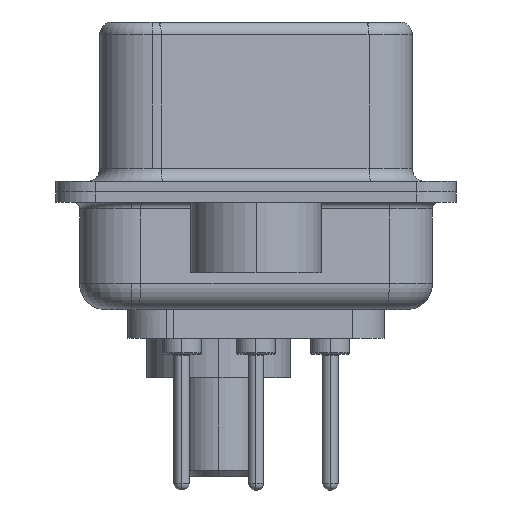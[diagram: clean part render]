
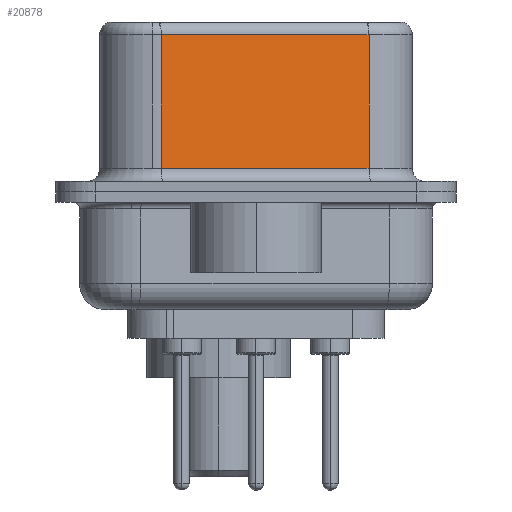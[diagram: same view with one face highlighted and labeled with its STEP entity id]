
A CAD part, left-side view. The second image highlights one B-rep face of the part: STEP entity #20878.
In plain terms, the highlighted planar face has unit normal (-0.985, -0.174, 0).
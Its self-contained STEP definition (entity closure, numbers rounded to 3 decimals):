
#35 = CARTESIAN_POINT ( 'NONE',  ( 5.132, -4.322, 0.9 ) ) ;
#919 = CARTESIAN_POINT ( 'NONE',  ( 5.132, -4.322, 6.52 ) ) ;
#1371 = LINE ( 'NONE', #1636, #23242 ) ;
#1636 = CARTESIAN_POINT ( 'NONE',  ( 5.132, -4.322, 6.02 ) ) ;
#1739 = VECTOR ( 'NONE', #6403, 1000. ) ;
#1904 = EDGE_CURVE ( 'NONE', #24573, #15131, #2415, .T. ) ;
#2415 = LINE ( 'NONE', #919, #1739 ) ;
#3811 = ORIENTED_EDGE ( 'NONE', *, *, #1904, .F. ) ;
#3835 = DIRECTION ( 'NONE',  ( -0.174, 0.985, 0. ) ) ;
#6403 = DIRECTION ( 'NONE',  ( 0., 0., -1. ) ) ;
#6709 = VERTEX_POINT ( 'NONE', #12838 ) ;
#6883 = CARTESIAN_POINT ( 'NONE',  ( 3.73, 3.628, 6.02 ) ) ;
#10946 = LINE ( 'NONE', #35, #27660 ) ;
#11010 = CARTESIAN_POINT ( 'NONE',  ( 3.73, 3.628, 6.52 ) ) ;
#11088 = CARTESIAN_POINT ( 'NONE',  ( 5.132, -4.322, 0.9 ) ) ;
#11819 = EDGE_CURVE ( 'NONE', #24573, #27920, #1371, .T. ) ;
#12649 = DIRECTION ( 'NONE',  ( 0.985, 0.174, 0. ) ) ;
#12838 = CARTESIAN_POINT ( 'NONE',  ( 3.73, 3.628, 0.9 ) ) ;
#13059 = LINE ( 'NONE', #11010, #23986 ) ;
#15131 = VERTEX_POINT ( 'NONE', #11088 ) ;
#17883 = EDGE_LOOP ( 'NONE', ( #3811, #19255, #24716, #22325 ) ) ;
#19084 = EDGE_CURVE ( 'NONE', #27920, #6709, #13059, .T. ) ;
#19255 = ORIENTED_EDGE ( 'NONE', *, *, #11819, .T. ) ;
#19712 = DIRECTION ( 'NONE',  ( 0., 0., -1. ) ) ;
#20878 = ADVANCED_FACE ( 'NONE', ( #22548 ), #23600, .F. ) ;
#21446 = CARTESIAN_POINT ( 'NONE',  ( 5.132, -4.322, 6.52 ) ) ;
#22028 = DIRECTION ( 'NONE',  ( 0.174, -0.985, 0. ) ) ;
#22325 = ORIENTED_EDGE ( 'NONE', *, *, #26611, .T. ) ;
#22548 = FACE_OUTER_BOUND ( 'NONE', #17883, .T. ) ;
#23242 = VECTOR ( 'NONE', #3835, 1000. ) ;
#23600 = PLANE ( 'NONE',  #27107 ) ;
#23986 = VECTOR ( 'NONE', #19712, 1000. ) ;
#24573 = VERTEX_POINT ( 'NONE', #25239 ) ;
#24716 = ORIENTED_EDGE ( 'NONE', *, *, #19084, .T. ) ;
#25239 = CARTESIAN_POINT ( 'NONE',  ( 5.132, -4.322, 6.02 ) ) ;
#25771 = DIRECTION ( 'NONE',  ( -0.174, 0.985, 0. ) ) ;
#26611 = EDGE_CURVE ( 'NONE', #6709, #15131, #10946, .T. ) ;
#27107 = AXIS2_PLACEMENT_3D ( 'NONE', #21446, #12649, #25771 ) ;
#27660 = VECTOR ( 'NONE', #22028, 1000. ) ;
#27920 = VERTEX_POINT ( 'NONE', #6883 ) ;
